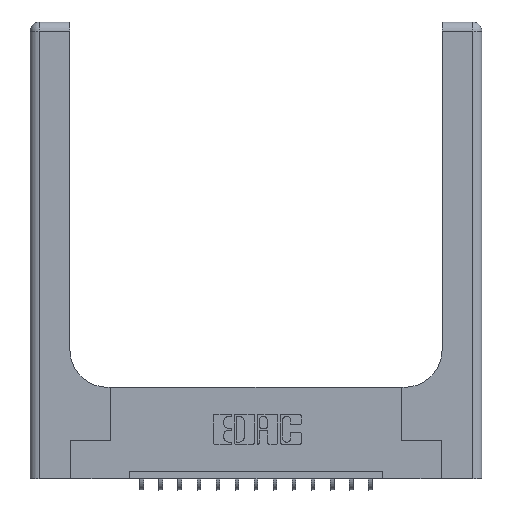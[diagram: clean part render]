
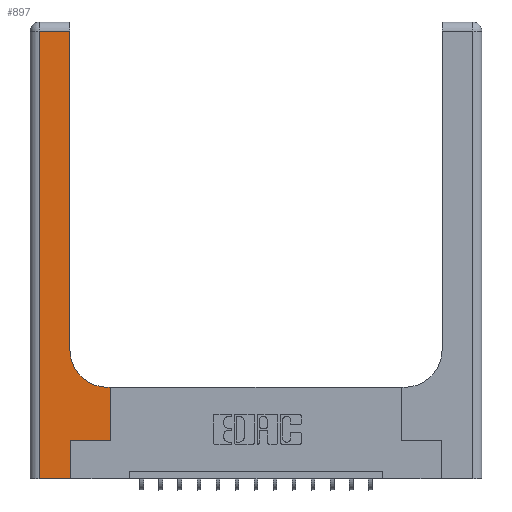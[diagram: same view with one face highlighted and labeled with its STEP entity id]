
A CAD part, top view. The second image highlights one B-rep face of the part: STEP entity #897.
In plain terms, the highlighted planar face has unit normal (0, 0, 1).
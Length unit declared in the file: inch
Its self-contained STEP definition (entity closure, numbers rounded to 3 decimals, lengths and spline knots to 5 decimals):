
#280 = EDGE_CURVE ( 'NONE', #6538, #6230, #11838, .T. ) ;
#591 = VECTOR ( 'NONE', #13585, 39.37008 ) ;
#673 = DIRECTION ( 'NONE',  ( 0., 0., -1. ) ) ;
#785 = EDGE_LOOP ( 'NONE', ( #6172, #4724, #8094, #4240, #2522, #9300, #2262, #9348, #12496 ) ) ;
#836 = VECTOR ( 'NONE', #10008, 39.37008 ) ;
#897 = ADVANCED_FACE ( 'NONE', ( #3361 ), #10333, .F. ) ;
#1505 = VERTEX_POINT ( 'NONE', #9992 ) ;
#1570 = DIRECTION ( 'NONE',  ( 1., 0., 0. ) ) ;
#1947 = VERTEX_POINT ( 'NONE', #14123 ) ;
#2111 = EDGE_CURVE ( 'NONE', #15330, #2906, #8234, .T. ) ;
#2262 = ORIENTED_EDGE ( 'NONE', *, *, #2111, .T. ) ;
#2522 = ORIENTED_EDGE ( 'NONE', *, *, #3073, .T. ) ;
#2707 = LINE ( 'NONE', #13590, #6496 ) ;
#2906 = VERTEX_POINT ( 'NONE', #16820 ) ;
#2998 = DIRECTION ( 'NONE',  ( -1., 0., 0. ) ) ;
#3073 = EDGE_CURVE ( 'NONE', #8377, #14731, #9578, .T. ) ;
#3258 = CARTESIAN_POINT ( 'NONE',  ( 0.528, 0.25, 0.37 ) ) ;
#3361 = FACE_OUTER_BOUND ( 'NONE', #785, .T. ) ;
#3680 = VECTOR ( 'NONE', #3981, 39.37008 ) ;
#3722 = EDGE_CURVE ( 'NONE', #1505, #11831, #12940, .T. ) ;
#3981 = DIRECTION ( 'NONE',  ( 0., 1., 0. ) ) ;
#4150 = AXIS2_PLACEMENT_3D ( 'NONE', #16751, #15492, #16850 ) ;
#4240 = ORIENTED_EDGE ( 'NONE', *, *, #4464, .T. ) ;
#4248 = CARTESIAN_POINT ( 'NONE',  ( 0.51, 0.6, 0.37 ) ) ;
#4464 = EDGE_CURVE ( 'NONE', #11831, #8377, #9783, .T. ) ;
#4724 = ORIENTED_EDGE ( 'NONE', *, *, #7777, .T. ) ;
#5502 = DIRECTION ( 'NONE',  ( 0., 1., 0. ) ) ;
#5513 = CARTESIAN_POINT ( 'NONE',  ( 0.26, 0.85, 0.37 ) ) ;
#5521 = LINE ( 'NONE', #6933, #12294 ) ;
#6018 = CARTESIAN_POINT ( 'NONE',  ( 0.265, 0.25, 0.37 ) ) ;
#6132 = DIRECTION ( 'NONE',  ( -1., 0., 0. ) ) ;
#6172 = ORIENTED_EDGE ( 'NONE', *, *, #12773, .T. ) ;
#6230 = VERTEX_POINT ( 'NONE', #5513 ) ;
#6496 = VECTOR ( 'NONE', #5502, 39.37008 ) ;
#6538 = VERTEX_POINT ( 'NONE', #4248 ) ;
#6933 = CARTESIAN_POINT ( 'NONE',  ( 0.26, 0.6, 0.37 ) ) ;
#7777 = EDGE_CURVE ( 'NONE', #1947, #1505, #8145, .T. ) ;
#8094 = ORIENTED_EDGE ( 'NONE', *, *, #3722, .T. ) ;
#8145 = LINE ( 'NONE', #12354, #591 ) ;
#8234 = LINE ( 'NONE', #8404, #9610 ) ;
#8377 = VERTEX_POINT ( 'NONE', #9112 ) ;
#8404 = CARTESIAN_POINT ( 'NONE',  ( 0.528, 0.25, 0.37 ) ) ;
#9112 = CARTESIAN_POINT ( 'NONE',  ( 0.265, 0., 0.37 ) ) ;
#9300 = ORIENTED_EDGE ( 'NONE', *, *, #10095, .T. ) ;
#9348 = ORIENTED_EDGE ( 'NONE', *, *, #12304, .T. ) ;
#9578 = LINE ( 'NONE', #16172, #3680 ) ;
#9610 = VECTOR ( 'NONE', #11185, 39.37008 ) ;
#9783 = LINE ( 'NONE', #9874, #15364 ) ;
#9874 = CARTESIAN_POINT ( 'NONE',  ( 0., 0., 0.37 ) ) ;
#9992 = CARTESIAN_POINT ( 'NONE',  ( 0.06, 2.94, 0.37 ) ) ;
#10008 = DIRECTION ( 'NONE',  ( 0., -1., 0. ) ) ;
#10095 = EDGE_CURVE ( 'NONE', #14731, #15330, #17161, .T. ) ;
#10333 = PLANE ( 'NONE',  #16938 ) ;
#10465 = CARTESIAN_POINT ( 'NONE',  ( 0.06, 0., 0.37 ) ) ;
#11185 = DIRECTION ( 'NONE',  ( 0., 1., 0. ) ) ;
#11794 = CARTESIAN_POINT ( 'NONE',  ( 0.06, 3., 0.37 ) ) ;
#11831 = VERTEX_POINT ( 'NONE', #10465 ) ;
#11838 = CIRCLE ( 'NONE', #4150, 0.25 ) ;
#12294 = VECTOR ( 'NONE', #2998, 39.37008 ) ;
#12304 = EDGE_CURVE ( 'NONE', #2906, #6538, #5521, .T. ) ;
#12354 = CARTESIAN_POINT ( 'NONE',  ( 0., 2.94, 0.37 ) ) ;
#12496 = ORIENTED_EDGE ( 'NONE', *, *, #280, .T. ) ;
#12773 = EDGE_CURVE ( 'NONE', #6230, #1947, #2707, .T. ) ;
#12900 = CARTESIAN_POINT ( 'NONE',  ( 0., 3., 0.37 ) ) ;
#12940 = LINE ( 'NONE', #11794, #836 ) ;
#13585 = DIRECTION ( 'NONE',  ( -1., 0., 0. ) ) ;
#13590 = CARTESIAN_POINT ( 'NONE',  ( 0.26, 3., 0.37 ) ) ;
#14123 = CARTESIAN_POINT ( 'NONE',  ( 0.26, 2.94, 0.37 ) ) ;
#14189 = DIRECTION ( 'NONE',  ( 1., 0., 0. ) ) ;
#14269 = CARTESIAN_POINT ( 'NONE',  ( 0.265, 0.25, 0.37 ) ) ;
#14731 = VERTEX_POINT ( 'NONE', #14269 ) ;
#15330 = VERTEX_POINT ( 'NONE', #3258 ) ;
#15364 = VECTOR ( 'NONE', #1570, 39.37008 ) ;
#15492 = DIRECTION ( 'NONE',  ( 0., 0., -1. ) ) ;
#16097 = VECTOR ( 'NONE', #14189, 39.37008 ) ;
#16172 = CARTESIAN_POINT ( 'NONE',  ( 0.265, 0., 0.37 ) ) ;
#16751 = CARTESIAN_POINT ( 'NONE',  ( 0.51, 0.85, 0.37 ) ) ;
#16820 = CARTESIAN_POINT ( 'NONE',  ( 0.528, 0.6, 0.37 ) ) ;
#16850 = DIRECTION ( 'NONE',  ( 1., 0., 0. ) ) ;
#16938 = AXIS2_PLACEMENT_3D ( 'NONE', #12900, #673, #6132 ) ;
#17161 = LINE ( 'NONE', #6018, #16097 ) ;
